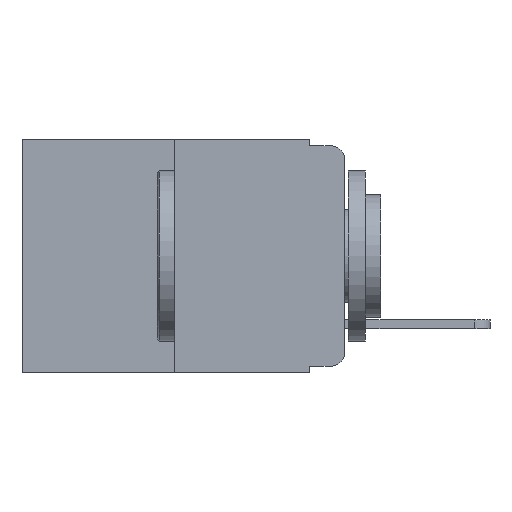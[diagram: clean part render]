
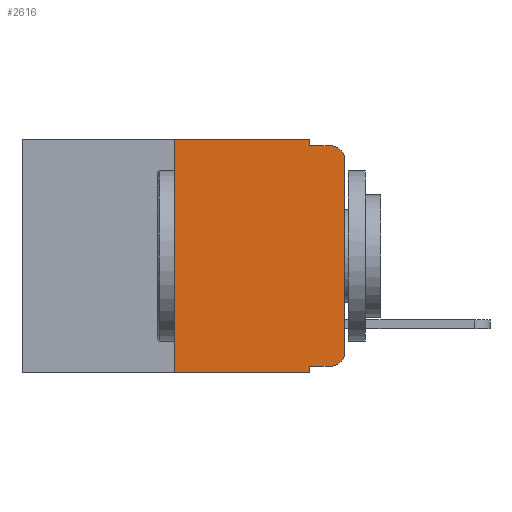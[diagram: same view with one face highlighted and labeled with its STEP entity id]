
A CAD part, left-side view. The second image highlights one B-rep face of the part: STEP entity #2616.
In plain terms, the highlighted planar face has unit normal (-1, 0, 0).
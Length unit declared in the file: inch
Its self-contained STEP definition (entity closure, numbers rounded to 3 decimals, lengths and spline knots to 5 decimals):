
#114 = VERTEX_POINT ( 'NONE', #2843 ) ;
#240 = EDGE_CURVE ( 'NONE', #4091, #3376, #14230, .T. ) ;
#342 = EDGE_CURVE ( 'NONE', #368, #3104, #6537, .T. ) ;
#349 = VECTOR ( 'NONE', #15402, 39.37008 ) ;
#368 = VERTEX_POINT ( 'NONE', #14881 ) ;
#556 = EDGE_CURVE ( 'NONE', #3422, #4091, #3171, .T. ) ;
#892 = AXIS2_PLACEMENT_3D ( 'NONE', #4688, #10731, #3885 ) ;
#1012 = VERTEX_POINT ( 'NONE', #4596 ) ;
#1981 = CARTESIAN_POINT ( 'NONE',  ( 0., 0.051, 0. ) ) ;
#2011 = ORIENTED_EDGE ( 'NONE', *, *, #10614, .F. ) ;
#2110 = VECTOR ( 'NONE', #13658, 39.37008 ) ;
#2469 = CARTESIAN_POINT ( 'NONE',  ( 0., 0.02, -0.333 ) ) ;
#2616 = ADVANCED_FACE ( 'NONE', ( #10474 ), #6549, .F. ) ;
#2686 = CARTESIAN_POINT ( 'NONE',  ( 0., 0.02, -0.01 ) ) ;
#2843 = CARTESIAN_POINT ( 'NONE',  ( 0., 0.051, -0.343 ) ) ;
#3081 = VERTEX_POINT ( 'NONE', #3410 ) ;
#3104 = VERTEX_POINT ( 'NONE', #2686 ) ;
#3147 = VECTOR ( 'NONE', #9598, 39.37008 ) ;
#3171 = LINE ( 'NONE', #8089, #12779 ) ;
#3303 = CARTESIAN_POINT ( 'NONE',  ( 0., 0.02, -0.03 ) ) ;
#3376 = VERTEX_POINT ( 'NONE', #14153 ) ;
#3410 = CARTESIAN_POINT ( 'NONE',  ( 0., 0.25, -0.343 ) ) ;
#3422 = VERTEX_POINT ( 'NONE', #12995 ) ;
#3729 = CARTESIAN_POINT ( 'NONE',  ( 0., 0.473, 0. ) ) ;
#3885 = DIRECTION ( 'NONE',  ( 0., 0., -1. ) ) ;
#3946 = VERTEX_POINT ( 'NONE', #1981 ) ;
#4091 = VERTEX_POINT ( 'NONE', #2469 ) ;
#4251 = EDGE_LOOP ( 'NONE', ( #15108, #9552, #8581, #6870, #7629, #14029, #11255, #2011, #14749, #12028 ) ) ;
#4540 = DIRECTION ( 'NONE',  ( 0., 0., -1. ) ) ;
#4596 = CARTESIAN_POINT ( 'NONE',  ( 0., 0., -0.03 ) ) ;
#4688 = CARTESIAN_POINT ( 'NONE',  ( 0., 0.02, -0.313 ) ) ;
#4856 = DIRECTION ( 'NONE',  ( 0., -1., 0. ) ) ;
#5222 = CARTESIAN_POINT ( 'NONE',  ( 0., 0.051, 0. ) ) ;
#5288 = EDGE_CURVE ( 'NONE', #7100, #3946, #6679, .T. ) ;
#5384 = LINE ( 'NONE', #8424, #11407 ) ;
#5660 = AXIS2_PLACEMENT_3D ( 'NONE', #3303, #11735, #4540 ) ;
#5771 = DIRECTION ( 'NONE',  ( 0., -1., 0. ) ) ;
#5796 = AXIS2_PLACEMENT_3D ( 'NONE', #7366, #14213, #9965 ) ;
#5976 = EDGE_CURVE ( 'NONE', #3081, #114, #6328, .T. ) ;
#6025 = DIRECTION ( 'NONE',  ( 0., 0., -1. ) ) ;
#6328 = LINE ( 'NONE', #14919, #3147 ) ;
#6537 = LINE ( 'NONE', #15500, #12610 ) ;
#6549 = PLANE ( 'NONE',  #5796 ) ;
#6679 = LINE ( 'NONE', #3729, #12752 ) ;
#6870 = ORIENTED_EDGE ( 'NONE', *, *, #8444, .F. ) ;
#7012 = CARTESIAN_POINT ( 'NONE',  ( 0., 0., 0. ) ) ;
#7100 = VERTEX_POINT ( 'NONE', #15244 ) ;
#7366 = CARTESIAN_POINT ( 'NONE',  ( 0., 0.473, 0. ) ) ;
#7629 = ORIENTED_EDGE ( 'NONE', *, *, #5288, .F. ) ;
#8089 = CARTESIAN_POINT ( 'NONE',  ( 0., 0.051, -0.333 ) ) ;
#8235 = CARTESIAN_POINT ( 'NONE',  ( 0., 0.25, 0. ) ) ;
#8359 = CIRCLE ( 'NONE', #5660, 0.02 ) ;
#8424 = CARTESIAN_POINT ( 'NONE',  ( 0., 0.051, 0. ) ) ;
#8444 = EDGE_CURVE ( 'NONE', #3946, #368, #8883, .T. ) ;
#8581 = ORIENTED_EDGE ( 'NONE', *, *, #342, .F. ) ;
#8883 = LINE ( 'NONE', #5222, #2110 ) ;
#9552 = ORIENTED_EDGE ( 'NONE', *, *, #10412, .T. ) ;
#9598 = DIRECTION ( 'NONE',  ( 0., -1., 0. ) ) ;
#9887 = EDGE_CURVE ( 'NONE', #3376, #1012, #13540, .T. ) ;
#9965 = DIRECTION ( 'NONE',  ( 0., 0., -1. ) ) ;
#10371 = VECTOR ( 'NONE', #14225, 39.37008 ) ;
#10412 = EDGE_CURVE ( 'NONE', #1012, #3104, #8359, .T. ) ;
#10474 = FACE_OUTER_BOUND ( 'NONE', #4251, .T. ) ;
#10614 = EDGE_CURVE ( 'NONE', #3422, #114, #5384, .T. ) ;
#10731 = DIRECTION ( 'NONE',  ( -1., 0., 0. ) ) ;
#11255 = ORIENTED_EDGE ( 'NONE', *, *, #5976, .T. ) ;
#11407 = VECTOR ( 'NONE', #6025, 39.37008 ) ;
#11735 = DIRECTION ( 'NONE',  ( -1., 0., 0. ) ) ;
#12028 = ORIENTED_EDGE ( 'NONE', *, *, #240, .T. ) ;
#12610 = VECTOR ( 'NONE', #15042, 39.37008 ) ;
#12752 = VECTOR ( 'NONE', #5771, 39.37008 ) ;
#12779 = VECTOR ( 'NONE', #4856, 39.37008 ) ;
#12995 = CARTESIAN_POINT ( 'NONE',  ( 0., 0.051, -0.333 ) ) ;
#13207 = LINE ( 'NONE', #8235, #349 ) ;
#13297 = EDGE_CURVE ( 'NONE', #3081, #7100, #13207, .T. ) ;
#13540 = LINE ( 'NONE', #7012, #10371 ) ;
#13658 = DIRECTION ( 'NONE',  ( 0., 0., -1. ) ) ;
#14029 = ORIENTED_EDGE ( 'NONE', *, *, #13297, .F. ) ;
#14153 = CARTESIAN_POINT ( 'NONE',  ( 0., 0., -0.313 ) ) ;
#14213 = DIRECTION ( 'NONE',  ( 1., 0., 0. ) ) ;
#14225 = DIRECTION ( 'NONE',  ( 0., 0., 1. ) ) ;
#14230 = CIRCLE ( 'NONE', #892, 0.02 ) ;
#14749 = ORIENTED_EDGE ( 'NONE', *, *, #556, .T. ) ;
#14881 = CARTESIAN_POINT ( 'NONE',  ( 0., 0.051, -0.01 ) ) ;
#14919 = CARTESIAN_POINT ( 'NONE',  ( 0., 0.473, -0.343 ) ) ;
#15042 = DIRECTION ( 'NONE',  ( 0., -1., 0. ) ) ;
#15108 = ORIENTED_EDGE ( 'NONE', *, *, #9887, .T. ) ;
#15244 = CARTESIAN_POINT ( 'NONE',  ( 0., 0.25, 0. ) ) ;
#15402 = DIRECTION ( 'NONE',  ( 0., 0., 1. ) ) ;
#15500 = CARTESIAN_POINT ( 'NONE',  ( 0., 0.051, -0.01 ) ) ;
